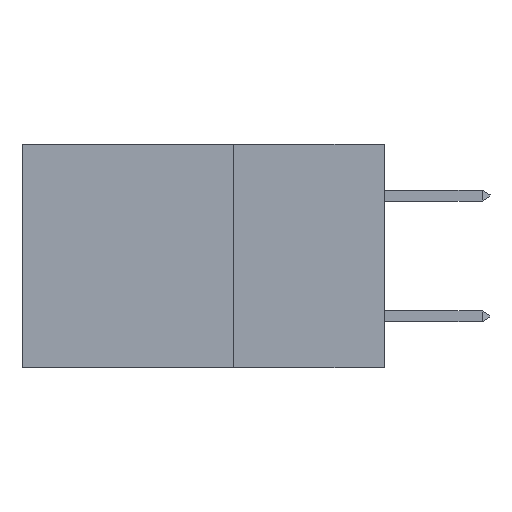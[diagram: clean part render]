
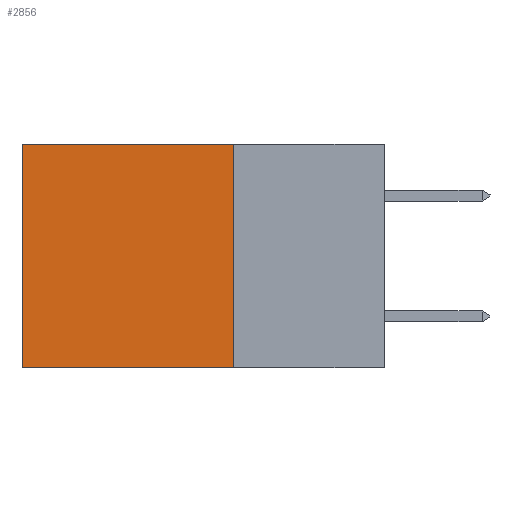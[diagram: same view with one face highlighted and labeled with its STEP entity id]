
A CAD part, left-side view. The second image highlights one B-rep face of the part: STEP entity #2856.
In plain terms, the highlighted planar face has unit normal (-1, 0, 0).
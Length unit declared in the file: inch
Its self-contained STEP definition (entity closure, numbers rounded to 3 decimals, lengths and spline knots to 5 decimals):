
#31 = EDGE_CURVE ( 'NONE', #9013, #8274, #12161, .T. ) ;
#1052 = VECTOR ( 'NONE', #13454, 39.37008 ) ;
#1133 = DIRECTION ( 'NONE',  ( 0., 1., 0. ) ) ;
#1584 = CARTESIAN_POINT ( 'NONE',  ( 0.2875, 0.25, 0. ) ) ;
#1975 = EDGE_CURVE ( 'NONE', #3518, #4856, #4587, .T. ) ;
#2627 = CARTESIAN_POINT ( 'NONE',  ( 0.2875, 0.6, 0. ) ) ;
#2856 = ADVANCED_FACE ( 'NONE', ( #11612 ), #10647, .F. ) ;
#3518 = VERTEX_POINT ( 'NONE', #9886 ) ;
#3689 = VECTOR ( 'NONE', #7387, 39.37008 ) ;
#3776 = AXIS2_PLACEMENT_3D ( 'NONE', #8547, #4329, #11662 ) ;
#3849 = VECTOR ( 'NONE', #12011, 39.37008 ) ;
#4030 = LINE ( 'NONE', #8409, #3689 ) ;
#4200 = EDGE_CURVE ( 'NONE', #9013, #3518, #12216, .T. ) ;
#4329 = DIRECTION ( 'NONE',  ( 1., 0., 0. ) ) ;
#4587 = LINE ( 'NONE', #6582, #12265 ) ;
#4754 = CARTESIAN_POINT ( 'NONE',  ( 0.2875, 0.25, 0. ) ) ;
#4856 = VERTEX_POINT ( 'NONE', #9890 ) ;
#5031 = ORIENTED_EDGE ( 'NONE', *, *, #10569, .T. ) ;
#5066 = ORIENTED_EDGE ( 'NONE', *, *, #1975, .F. ) ;
#5115 = ORIENTED_EDGE ( 'NONE', *, *, #4200, .F. ) ;
#5152 = ORIENTED_EDGE ( 'NONE', *, *, #31, .T. ) ;
#6582 = CARTESIAN_POINT ( 'NONE',  ( 0.2875, 0.25, -0.37 ) ) ;
#7387 = DIRECTION ( 'NONE',  ( 0., 0., -1. ) ) ;
#8274 = VERTEX_POINT ( 'NONE', #2627 ) ;
#8409 = CARTESIAN_POINT ( 'NONE',  ( 0.2875, 0.6, 0. ) ) ;
#8547 = CARTESIAN_POINT ( 'NONE',  ( 0.2875, 0.25, 0. ) ) ;
#8553 = CARTESIAN_POINT ( 'NONE',  ( 0.2875, 0.25, 0. ) ) ;
#8903 = EDGE_LOOP ( 'NONE', ( #5031, #5066, #5115, #5152 ) ) ;
#9013 = VERTEX_POINT ( 'NONE', #1584 ) ;
#9886 = CARTESIAN_POINT ( 'NONE',  ( 0.2875, 0.25, -0.37 ) ) ;
#9890 = CARTESIAN_POINT ( 'NONE',  ( 0.2875, 0.6, -0.37 ) ) ;
#10569 = EDGE_CURVE ( 'NONE', #8274, #4856, #4030, .T. ) ;
#10647 = PLANE ( 'NONE',  #3776 ) ;
#11612 = FACE_OUTER_BOUND ( 'NONE', #8903, .T. ) ;
#11662 = DIRECTION ( 'NONE',  ( 0., 0., -1. ) ) ;
#12011 = DIRECTION ( 'NONE',  ( 0., 0., -1. ) ) ;
#12161 = LINE ( 'NONE', #8553, #1052 ) ;
#12216 = LINE ( 'NONE', #4754, #3849 ) ;
#12265 = VECTOR ( 'NONE', #1133, 39.37008 ) ;
#13454 = DIRECTION ( 'NONE',  ( 0., 1., 0. ) ) ;
